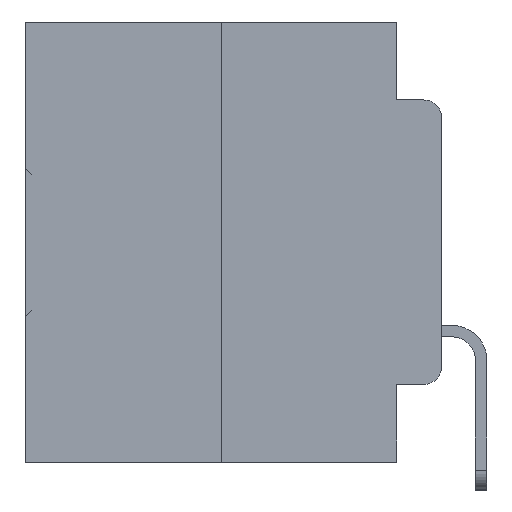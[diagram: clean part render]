
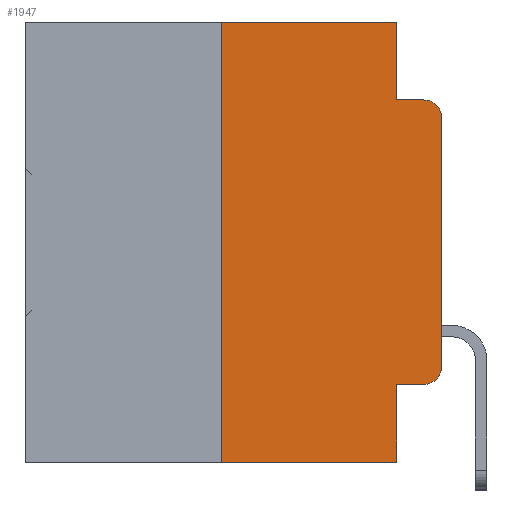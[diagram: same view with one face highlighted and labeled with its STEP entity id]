
A CAD part, left-side view. The second image highlights one B-rep face of the part: STEP entity #1947.
In plain terms, the highlighted planar face has unit normal (-1, 0, 0).
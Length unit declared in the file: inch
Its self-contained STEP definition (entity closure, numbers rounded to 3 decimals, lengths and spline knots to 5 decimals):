
#64 = ORIENTED_EDGE ( 'NONE', *, *, #921, .F. ) ;
#147 = ORIENTED_EDGE ( 'NONE', *, *, #18882, .T. ) ;
#284 = ORIENTED_EDGE ( 'NONE', *, *, #21068, .F. ) ;
#862 = DIRECTION ( 'NONE',  ( -1., 0., 0. ) ) ;
#921 = EDGE_CURVE ( 'NONE', #30913, #33824, #7146, .T. ) ;
#1254 = ORIENTED_EDGE ( 'NONE', *, *, #6875, .F. ) ;
#1827 = CARTESIAN_POINT ( 'NONE',  ( 0., 0.25, 0. ) ) ;
#1947 = ADVANCED_FACE ( 'NONE', ( #21928 ), #12950, .F. ) ;
#2248 = CIRCLE ( 'NONE', #12843, 0.02 ) ;
#2893 = DIRECTION ( 'NONE',  ( 0., -1., 0. ) ) ;
#2947 = ORIENTED_EDGE ( 'NONE', *, *, #28613, .T. ) ;
#3216 = CARTESIAN_POINT ( 'NONE',  ( 0., 0., 0. ) ) ;
#3620 = EDGE_CURVE ( 'NONE', #33824, #28185, #5272, .T. ) ;
#3636 = CARTESIAN_POINT ( 'NONE',  ( 0., 0.25, -0.5 ) ) ;
#4353 = ORIENTED_EDGE ( 'NONE', *, *, #29641, .T. ) ;
#4536 = VERTEX_POINT ( 'NONE', #7187 ) ;
#4685 = CARTESIAN_POINT ( 'NONE',  ( 0., 0.02, -0.4115 ) ) ;
#5264 = CARTESIAN_POINT ( 'NONE',  ( 0., 0.02, -0.0885 ) ) ;
#5272 = LINE ( 'NONE', #24224, #24050 ) ;
#5622 = DIRECTION ( 'NONE',  ( 0., -1., 0. ) ) ;
#5923 = CARTESIAN_POINT ( 'NONE',  ( 0., 0.473, -0.5 ) ) ;
#6033 = CIRCLE ( 'NONE', #31314, 0.02 ) ;
#6236 = DIRECTION ( 'NONE',  ( 0., 0., 1. ) ) ;
#6259 = ORIENTED_EDGE ( 'NONE', *, *, #22138, .T. ) ;
#6372 = VECTOR ( 'NONE', #22217, 39.37008 ) ;
#6875 = EDGE_CURVE ( 'NONE', #17298, #33678, #13657, .T. ) ;
#6939 = ORIENTED_EDGE ( 'NONE', *, *, #12387, .F. ) ;
#6972 = ORIENTED_EDGE ( 'NONE', *, *, #30258, .T. ) ;
#7118 = LINE ( 'NONE', #14136, #33125 ) ;
#7146 = LINE ( 'NONE', #26257, #25659 ) ;
#7187 = CARTESIAN_POINT ( 'NONE',  ( 0., 0.051, -0.0885 ) ) ;
#7818 = VERTEX_POINT ( 'NONE', #4685 ) ;
#8134 = VECTOR ( 'NONE', #8775, 39.37008 ) ;
#8775 = DIRECTION ( 'NONE',  ( 0., -1., 0. ) ) ;
#9657 = VERTEX_POINT ( 'NONE', #27633 ) ;
#9897 = DIRECTION ( 'NONE',  ( -1., 0., 0. ) ) ;
#10093 = CARTESIAN_POINT ( 'NONE',  ( 0., 0.051, 0. ) ) ;
#10487 = VECTOR ( 'NONE', #32058, 39.37008 ) ;
#10675 = LINE ( 'NONE', #5923, #8134 ) ;
#10889 = VERTEX_POINT ( 'NONE', #32706 ) ;
#12387 = EDGE_CURVE ( 'NONE', #4536, #13202, #26486, .T. ) ;
#12473 = CARTESIAN_POINT ( 'NONE',  ( 0., 0.473, 0. ) ) ;
#12843 = AXIS2_PLACEMENT_3D ( 'NONE', #17469, #862, #20026 ) ;
#12950 = PLANE ( 'NONE',  #15399 ) ;
#13202 = VERTEX_POINT ( 'NONE', #5264 ) ;
#13657 = LINE ( 'NONE', #29766, #6372 ) ;
#13810 = VECTOR ( 'NONE', #6236, 39.37008 ) ;
#14136 = CARTESIAN_POINT ( 'NONE',  ( 0., 0.051, 0. ) ) ;
#14180 = ORIENTED_EDGE ( 'NONE', *, *, #3620, .F. ) ;
#15399 = AXIS2_PLACEMENT_3D ( 'NONE', #12473, #16075, #15993 ) ;
#15993 = DIRECTION ( 'NONE',  ( 0., 0., -1. ) ) ;
#16075 = DIRECTION ( 'NONE',  ( 1., 0., 0. ) ) ;
#17298 = VERTEX_POINT ( 'NONE', #19879 ) ;
#17469 = CARTESIAN_POINT ( 'NONE',  ( 0., 0.02, -0.3915 ) ) ;
#18882 = EDGE_CURVE ( 'NONE', #30913, #33678, #10675, .T. ) ;
#19879 = CARTESIAN_POINT ( 'NONE',  ( 0., 0.051, -0.4115 ) ) ;
#20026 = DIRECTION ( 'NONE',  ( 0., 0., -1. ) ) ;
#21068 = EDGE_CURVE ( 'NONE', #28185, #4536, #7118, .T. ) ;
#21928 = FACE_OUTER_BOUND ( 'NONE', #32593, .T. ) ;
#22138 = EDGE_CURVE ( 'NONE', #10889, #9657, #34176, .T. ) ;
#22217 = DIRECTION ( 'NONE',  ( 0., 0., -1. ) ) ;
#24050 = VECTOR ( 'NONE', #5622, 39.37008 ) ;
#24224 = CARTESIAN_POINT ( 'NONE',  ( 0., 0.473, 0. ) ) ;
#24554 = DIRECTION ( 'NONE',  ( 0., 0., -1. ) ) ;
#24596 = CARTESIAN_POINT ( 'NONE',  ( 0., 0.051, -0.4115 ) ) ;
#25515 = CARTESIAN_POINT ( 'NONE',  ( 0., 0.02, -0.1085 ) ) ;
#25659 = VECTOR ( 'NONE', #26279, 39.37008 ) ;
#26257 = CARTESIAN_POINT ( 'NONE',  ( 0., 0.25, 0. ) ) ;
#26279 = DIRECTION ( 'NONE',  ( 0., 0., 1. ) ) ;
#26486 = LINE ( 'NONE', #29548, #32367 ) ;
#27633 = CARTESIAN_POINT ( 'NONE',  ( 0., 0., -0.1085 ) ) ;
#28068 = DIRECTION ( 'NONE',  ( 0., 0., -1. ) ) ;
#28185 = VERTEX_POINT ( 'NONE', #10093 ) ;
#28613 = EDGE_CURVE ( 'NONE', #17298, #7818, #31861, .T. ) ;
#29548 = CARTESIAN_POINT ( 'NONE',  ( 0., 0.051, -0.0885 ) ) ;
#29641 = EDGE_CURVE ( 'NONE', #9657, #13202, #6033, .T. ) ;
#29766 = CARTESIAN_POINT ( 'NONE',  ( 0., 0.051, 0. ) ) ;
#30258 = EDGE_CURVE ( 'NONE', #7818, #10889, #2248, .T. ) ;
#30381 = CARTESIAN_POINT ( 'NONE',  ( 0., 0.051, -0.5 ) ) ;
#30913 = VERTEX_POINT ( 'NONE', #3636 ) ;
#31314 = AXIS2_PLACEMENT_3D ( 'NONE', #25515, #9897, #28068 ) ;
#31861 = LINE ( 'NONE', #24596, #10487 ) ;
#32058 = DIRECTION ( 'NONE',  ( 0., -1., 0. ) ) ;
#32367 = VECTOR ( 'NONE', #2893, 39.37008 ) ;
#32593 = EDGE_LOOP ( 'NONE', ( #6259, #4353, #6939, #284, #14180, #64, #147, #1254, #2947, #6972 ) ) ;
#32706 = CARTESIAN_POINT ( 'NONE',  ( 0., 0., -0.3915 ) ) ;
#33125 = VECTOR ( 'NONE', #24554, 39.37008 ) ;
#33678 = VERTEX_POINT ( 'NONE', #30381 ) ;
#33824 = VERTEX_POINT ( 'NONE', #1827 ) ;
#34176 = LINE ( 'NONE', #3216, #13810 ) ;
